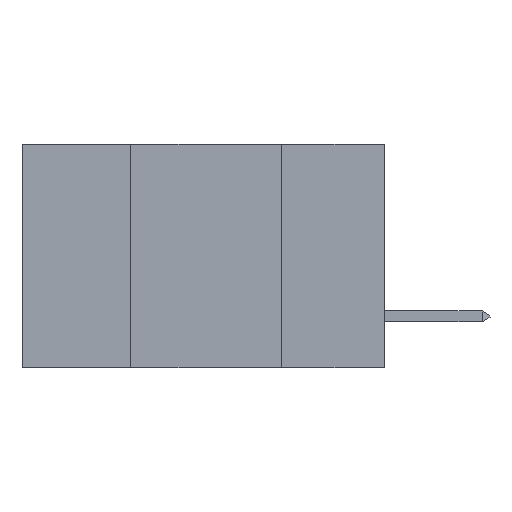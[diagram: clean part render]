
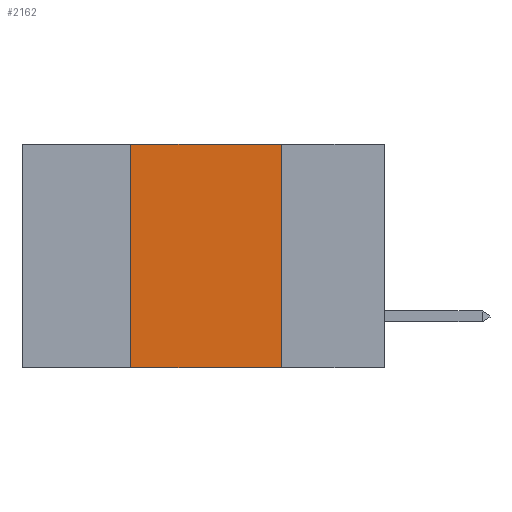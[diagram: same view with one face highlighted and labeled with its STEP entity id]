
A CAD part, left-side view. The second image highlights one B-rep face of the part: STEP entity #2162.
In plain terms, the highlighted planar face has unit normal (-1, 0, 0).
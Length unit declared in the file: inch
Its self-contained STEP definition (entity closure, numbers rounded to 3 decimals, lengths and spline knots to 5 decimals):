
#39 = LINE ( 'NONE', #8798, #10805 ) ;
#203 = VECTOR ( 'NONE', #13161, 39.37008 ) ;
#663 = LINE ( 'NONE', #11714, #203 ) ;
#1077 = DIRECTION ( 'NONE',  ( 0., -1., 0. ) ) ;
#1970 = AXIS2_PLACEMENT_3D ( 'NONE', #10243, #13191, #11347 ) ;
#2162 = ADVANCED_FACE ( 'NONE', ( #16324 ), #3881, .F. ) ;
#2332 = EDGE_CURVE ( 'NONE', #4675, #7901, #4521, .T. ) ;
#3324 = DIRECTION ( 'NONE',  ( 0., 0., -1. ) ) ;
#3881 = PLANE ( 'NONE',  #1970 ) ;
#4146 = VECTOR ( 'NONE', #1077, 39.37008 ) ;
#4353 = DIRECTION ( 'NONE',  ( 0., -1., 0. ) ) ;
#4521 = LINE ( 'NONE', #4698, #15638 ) ;
#4675 = VERTEX_POINT ( 'NONE', #8730 ) ;
#4698 = CARTESIAN_POINT ( 'NONE',  ( 0., 0.17, 0. ) ) ;
#5954 = EDGE_CURVE ( 'NONE', #8829, #4675, #8057, .T. ) ;
#6388 = CARTESIAN_POINT ( 'NONE',  ( 0., 0.42, 0. ) ) ;
#6663 = VERTEX_POINT ( 'NONE', #15964 ) ;
#7901 = VERTEX_POINT ( 'NONE', #10054 ) ;
#8057 = LINE ( 'NONE', #18476, #4146 ) ;
#8730 = CARTESIAN_POINT ( 'NONE',  ( 0., 0.17, 0. ) ) ;
#8798 = CARTESIAN_POINT ( 'NONE',  ( 0., 0.6, -0.37 ) ) ;
#8829 = VERTEX_POINT ( 'NONE', #6388 ) ;
#10054 = CARTESIAN_POINT ( 'NONE',  ( 0., 0.17, -0.37 ) ) ;
#10065 = EDGE_LOOP ( 'NONE', ( #16508, #12477, #11576, #10100 ) ) ;
#10100 = ORIENTED_EDGE ( 'NONE', *, *, #11754, .T. ) ;
#10243 = CARTESIAN_POINT ( 'NONE',  ( 0., 0.6, 0. ) ) ;
#10805 = VECTOR ( 'NONE', #4353, 39.37008 ) ;
#11347 = DIRECTION ( 'NONE',  ( 0., 0., -1. ) ) ;
#11576 = ORIENTED_EDGE ( 'NONE', *, *, #14289, .F. ) ;
#11714 = CARTESIAN_POINT ( 'NONE',  ( 0., 0.42, 0. ) ) ;
#11754 = EDGE_CURVE ( 'NONE', #6663, #7901, #39, .T. ) ;
#12477 = ORIENTED_EDGE ( 'NONE', *, *, #5954, .F. ) ;
#13161 = DIRECTION ( 'NONE',  ( 0., 0., 1. ) ) ;
#13191 = DIRECTION ( 'NONE',  ( 1., 0., 0. ) ) ;
#14289 = EDGE_CURVE ( 'NONE', #6663, #8829, #663, .T. ) ;
#15638 = VECTOR ( 'NONE', #3324, 39.37008 ) ;
#15964 = CARTESIAN_POINT ( 'NONE',  ( 0., 0.42, -0.37 ) ) ;
#16324 = FACE_OUTER_BOUND ( 'NONE', #10065, .T. ) ;
#16508 = ORIENTED_EDGE ( 'NONE', *, *, #2332, .F. ) ;
#18476 = CARTESIAN_POINT ( 'NONE',  ( 0., 0.6, 0. ) ) ;
